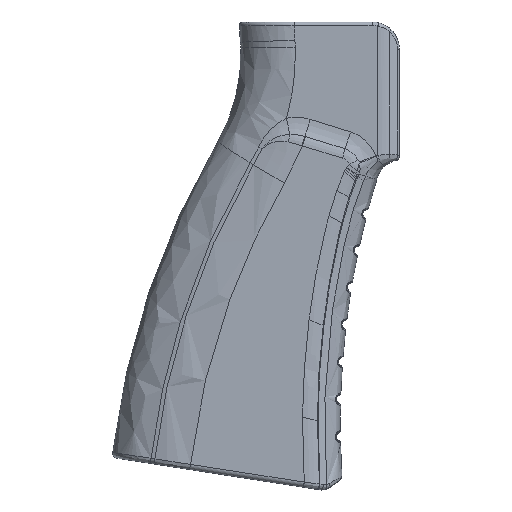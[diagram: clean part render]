
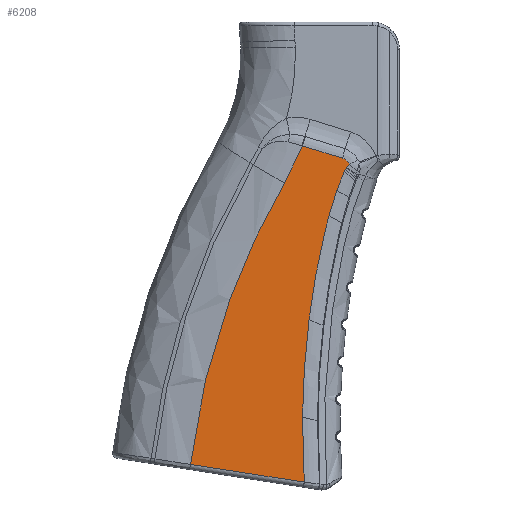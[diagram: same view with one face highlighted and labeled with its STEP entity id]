
A CAD part, left-side view. The second image highlights one B-rep face of the part: STEP entity #6208.
In plain terms, the highlighted planar face has unit normal (-1, 0, 0).
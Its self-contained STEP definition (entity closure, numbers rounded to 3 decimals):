
#621=B_SPLINE_CURVE_WITH_KNOTS('',3,(#18090,#18091,#18092,#18093,#18094),
 .UNSPECIFIED.,.F.,.F.,(4,1,4),(-6.95,-2.981,-0.008),
 .UNSPECIFIED.);
#625=B_SPLINE_CURVE_WITH_KNOTS('',3,(#18130,#18131,#18132,#18133,#18134,
#18135,#18136),.UNSPECIFIED.,.F.,.F.,(4,3,4),(-0.065,0.,1.429),
 .UNSPECIFIED.);
#626=B_SPLINE_CURVE_WITH_KNOTS('',3,(#18138,#18139,#18140,#18141),
 .UNSPECIFIED.,.F.,.F.,(4,4),(1.429,3.664),
 .UNSPECIFIED.);
#627=B_SPLINE_CURVE_WITH_KNOTS('',3,(#18143,#18144,#18145,#18146,#18147,
#18148),.UNSPECIFIED.,.F.,.F.,(4,2,4),(3.664,5.716,
5.716),.UNSPECIFIED.);
#628=B_SPLINE_CURVE_WITH_KNOTS('',3,(#18150,#18151,#18152,#18153),
 .UNSPECIFIED.,.F.,.F.,(4,4),(5.716,6.101),
 .UNSPECIFIED.);
#629=B_SPLINE_CURVE_WITH_KNOTS('',3,(#18155,#18156,#18157,#18158),
 .UNSPECIFIED.,.F.,.F.,(4,4),(6.101,6.711),
 .UNSPECIFIED.);
#630=B_SPLINE_CURVE_WITH_KNOTS('',3,(#18160,#18161,#18162,#18163),
 .UNSPECIFIED.,.F.,.F.,(4,4),(6.711,7.144),
 .UNSPECIFIED.);
#631=B_SPLINE_CURVE_WITH_KNOTS('',3,(#18165,#18166,#18167,#18168),
 .UNSPECIFIED.,.F.,.F.,(4,4),(7.144,7.197),
 .UNSPECIFIED.);
#632=B_SPLINE_CURVE_WITH_KNOTS('',3,(#18170,#18171,#18172,#18173),
 .UNSPECIFIED.,.F.,.F.,(4,4),(7.197,7.255),
 .UNSPECIFIED.);
#633=B_SPLINE_CURVE_WITH_KNOTS('',3,(#18180,#18181,#18182,#18183),
 .UNSPECIFIED.,.F.,.F.,(4,4),(-0.498,0.467),
 .UNSPECIFIED.);
#734=PLANE('',#6721);
#928=LINE('',#17782,#1140);
#930=LINE('',#18175,#1142);
#931=LINE('',#18179,#1143);
#1140=VECTOR('',#7809,10.);
#1142=VECTOR('',#7831,10.);
#1143=VECTOR('',#7834,10.);
#1588=FACE_OUTER_BOUND('',#2004,.T.);
#2004=EDGE_LOOP('',(#5482,#5483,#5484,#5485,#5486,#5487,#5488,#5489,#5490,
#5491,#5492,#5493,#5494,#5495));
#2354=CIRCLE('',#6722,2.695);
#2873=VERTEX_POINT('',#17771);
#2875=VERTEX_POINT('',#17780);
#2884=VERTEX_POINT('',#18089);
#2887=VERTEX_POINT('',#18129);
#2888=VERTEX_POINT('',#18137);
#2889=VERTEX_POINT('',#18142);
#2890=VERTEX_POINT('',#18149);
#2891=VERTEX_POINT('',#18154);
#2892=VERTEX_POINT('',#18159);
#2893=VERTEX_POINT('',#18164);
#2894=VERTEX_POINT('',#18169);
#2895=VERTEX_POINT('',#18174);
#2896=VERTEX_POINT('',#18176);
#2897=VERTEX_POINT('',#18178);
#3751=EDGE_CURVE('',#2873,#2875,#928,.T.);
#3771=EDGE_CURVE('',#2875,#2884,#621,.T.);
#3775=EDGE_CURVE('',#2873,#2887,#625,.T.);
#3776=EDGE_CURVE('',#2887,#2888,#626,.T.);
#3777=EDGE_CURVE('',#2888,#2889,#627,.T.);
#3778=EDGE_CURVE('',#2889,#2890,#628,.T.);
#3779=EDGE_CURVE('',#2890,#2891,#629,.T.);
#3780=EDGE_CURVE('',#2891,#2892,#630,.T.);
#3781=EDGE_CURVE('',#2892,#2893,#631,.T.);
#3782=EDGE_CURVE('',#2893,#2894,#632,.T.);
#3783=EDGE_CURVE('',#2895,#2894,#930,.T.);
#3784=EDGE_CURVE('',#2896,#2895,#2354,.T.);
#3785=EDGE_CURVE('',#2897,#2896,#931,.T.);
#3786=EDGE_CURVE('',#2884,#2897,#633,.T.);
#5482=ORIENTED_EDGE('',*,*,#3751,.F.);
#5483=ORIENTED_EDGE('',*,*,#3775,.T.);
#5484=ORIENTED_EDGE('',*,*,#3776,.T.);
#5485=ORIENTED_EDGE('',*,*,#3777,.T.);
#5486=ORIENTED_EDGE('',*,*,#3778,.T.);
#5487=ORIENTED_EDGE('',*,*,#3779,.T.);
#5488=ORIENTED_EDGE('',*,*,#3780,.T.);
#5489=ORIENTED_EDGE('',*,*,#3781,.T.);
#5490=ORIENTED_EDGE('',*,*,#3782,.T.);
#5491=ORIENTED_EDGE('',*,*,#3783,.F.);
#5492=ORIENTED_EDGE('',*,*,#3784,.F.);
#5493=ORIENTED_EDGE('',*,*,#3785,.F.);
#5494=ORIENTED_EDGE('',*,*,#3786,.F.);
#5495=ORIENTED_EDGE('',*,*,#3771,.F.);
#6208=ADVANCED_FACE('',(#1588),#734,.T.);
#6721=AXIS2_PLACEMENT_3D('',#18128,#7829,#7830);
#6722=AXIS2_PLACEMENT_3D('',#18177,#7832,#7833);
#7809=DIRECTION('',(0.,0.988,0.154));
#7829=DIRECTION('center_axis',(-1.,0.,0.));
#7830=DIRECTION('ref_axis',(0.,-1.,0.));
#7831=DIRECTION('',(0.,0.65,-0.76));
#7832=DIRECTION('center_axis',(1.,0.,0.));
#7833=DIRECTION('ref_axis',(0.,-0.599,0.801));
#7834=DIRECTION('',(0.,-0.955,-0.296));
#17771=CARTESIAN_POINT('',(-12.74,-132.168,-116.174));
#17780=CARTESIAN_POINT('',(-12.74,-105.732,-112.054));
#17782=CARTESIAN_POINT('',(-12.74,-108.052,-112.415));
#18089=CARTESIAN_POINT('',(-12.74,-127.571,-46.672));
#18090=CARTESIAN_POINT('Ctrl Pts',(-12.74,-105.732,
-112.054));
#18091=CARTESIAN_POINT('Ctrl Pts',(-12.74,-107.286,-98.917));
#18092=CARTESIAN_POINT('Ctrl Pts',(-12.74,-112.706,-76.259));
#18093=CARTESIAN_POINT('Ctrl Pts',(-12.74,-122.587,
-55.237));
#18094=CARTESIAN_POINT('Ctrl Pts',(-12.74,-127.571,
-46.672));
#18128=CARTESIAN_POINT('Origin',(-12.74,-124.662,-63.494));
#18129=CARTESIAN_POINT('',(-12.74,-131.769,-101.065));
#18130=CARTESIAN_POINT('Ctrl Pts',(-12.74,-132.168,-116.174));
#18131=CARTESIAN_POINT('Ctrl Pts',(-12.74,-132.154,-115.954));
#18132=CARTESIAN_POINT('Ctrl Pts',(-12.74,-132.141,-115.733));
#18133=CARTESIAN_POINT('Ctrl Pts',(-12.74,-132.127,-115.513));
#18134=CARTESIAN_POINT('Ctrl Pts',(-12.74,-131.837,
-110.702));
#18135=CARTESIAN_POINT('Ctrl Pts',(-12.74,-131.717,
-105.883));
#18136=CARTESIAN_POINT('Ctrl Pts',(-12.74,-131.769,-101.065));
#18137=CARTESIAN_POINT('',(-12.74,-133.268,-78.508));
#18138=CARTESIAN_POINT('Ctrl Pts',(-12.74,-131.769,-101.065));
#18139=CARTESIAN_POINT('Ctrl Pts',(-12.74,-131.849,
-93.527));
#18140=CARTESIAN_POINT('Ctrl Pts',(-12.74,-132.345,
-85.993));
#18141=CARTESIAN_POINT('Ctrl Pts',(-12.74,-133.268,-78.508));
#18142=CARTESIAN_POINT('',(-12.74,-136.957,-58.071));
#18143=CARTESIAN_POINT('Ctrl Pts',(-12.74,-133.268,-78.508));
#18144=CARTESIAN_POINT('Ctrl Pts',(-12.74,-134.115,
-71.642));
#18145=CARTESIAN_POINT('Ctrl Pts',(-12.74,-135.322,
-64.81));
#18146=CARTESIAN_POINT('Ctrl Pts',(-12.74,-136.957,
-58.071));
#18147=CARTESIAN_POINT('Ctrl Pts',(-12.74,-136.957,
-58.071));
#18148=CARTESIAN_POINT('Ctrl Pts',(-12.74,-136.957,
-58.071));
#18149=CARTESIAN_POINT('',(-12.74,-137.929,-54.279));
#18150=CARTESIAN_POINT('Ctrl Pts',(-12.74,-136.957,
-58.071));
#18151=CARTESIAN_POINT('Ctrl Pts',(-12.74,-137.265,
-56.804));
#18152=CARTESIAN_POINT('Ctrl Pts',(-12.74,-137.588,
-55.54));
#18153=CARTESIAN_POINT('Ctrl Pts',(-12.74,-137.929,
-54.279));
#18154=CARTESIAN_POINT('',(-12.74,-139.743,-48.299));
#18155=CARTESIAN_POINT('Ctrl Pts',(-12.74,-137.929,
-54.279));
#18156=CARTESIAN_POINT('Ctrl Pts',(-12.74,-138.466,
-52.289));
#18157=CARTESIAN_POINT('Ctrl Pts',(-12.74,-139.051,
-50.286));
#18158=CARTESIAN_POINT('Ctrl Pts',(-12.74,-139.743,
-48.299));
#18159=CARTESIAN_POINT('',(-12.74,-141.488,-44.063));
#18160=CARTESIAN_POINT('Ctrl Pts',(-12.74,-139.743,
-48.299));
#18161=CARTESIAN_POINT('Ctrl Pts',(-12.74,-140.236,-46.885));
#18162=CARTESIAN_POINT('Ctrl Pts',(-12.74,-140.797,
-45.456));
#18163=CARTESIAN_POINT('Ctrl Pts',(-12.74,-141.488,
-44.063));
#18164=CARTESIAN_POINT('',(-12.74,-141.744,-43.559));
#18165=CARTESIAN_POINT('Ctrl Pts',(-12.74,-141.488,
-44.063));
#18166=CARTESIAN_POINT('Ctrl Pts',(-12.74,-141.572,-43.893));
#18167=CARTESIAN_POINT('Ctrl Pts',(-12.74,-141.658,-43.725));
#18168=CARTESIAN_POINT('Ctrl Pts',(-12.74,-141.744,
-43.559));
#18169=CARTESIAN_POINT('',(-12.74,-142.034,-43.013));
#18170=CARTESIAN_POINT('Ctrl Pts',(-12.74,-141.744,
-43.559));
#18171=CARTESIAN_POINT('Ctrl Pts',(-12.74,-141.838,
-43.377));
#18172=CARTESIAN_POINT('Ctrl Pts',(-12.74,-141.935,
-43.194));
#18173=CARTESIAN_POINT('Ctrl Pts',(-12.74,-142.034,
-43.013));
#18174=CARTESIAN_POINT('',(-12.74,-142.662,-42.278));
#18175=CARTESIAN_POINT('',(-12.74,-142.034,-43.013));
#18176=CARTESIAN_POINT('',(-12.74,-141.03,-40.869));
#18177=CARTESIAN_POINT('Origin',(-12.74,-140.232,-43.443));
#18178=CARTESIAN_POINT('',(-12.74,-131.783,-38.004));
#18179=CARTESIAN_POINT('',(-12.74,-153.895,-44.857));
#18180=CARTESIAN_POINT('Ctrl Pts',(-12.74,-127.571,
-46.672));
#18181=CARTESIAN_POINT('Ctrl Pts',(-12.74,-129.211,
-43.905));
#18182=CARTESIAN_POINT('Ctrl Pts',(-12.74,-130.621,
-41.003));
#18183=CARTESIAN_POINT('Ctrl Pts',(-12.74,-131.783,
-38.004));
